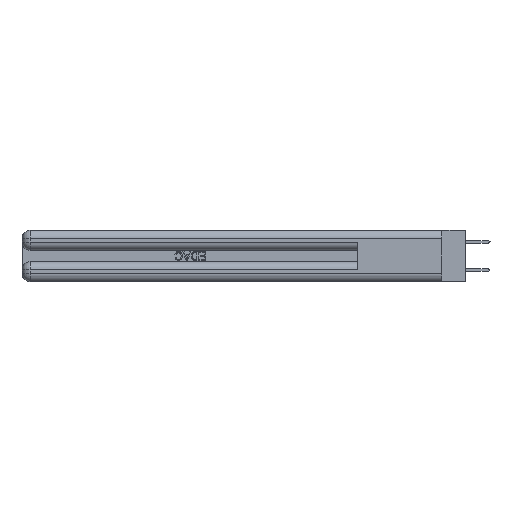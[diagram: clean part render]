
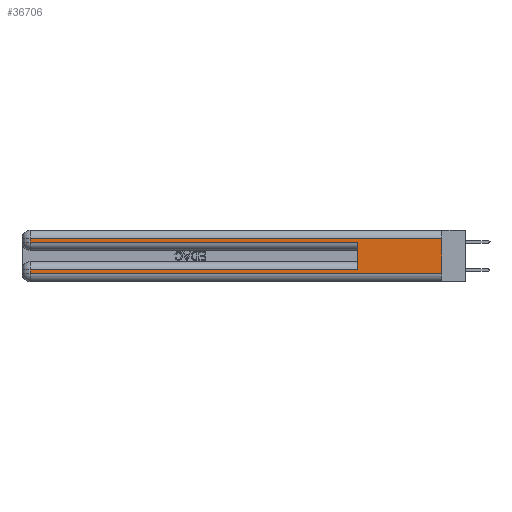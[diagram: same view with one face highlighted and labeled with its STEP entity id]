
A CAD part, left-side view. The second image highlights one B-rep face of the part: STEP entity #36706.
In plain terms, the highlighted planar face has unit normal (-1, 0, 0).
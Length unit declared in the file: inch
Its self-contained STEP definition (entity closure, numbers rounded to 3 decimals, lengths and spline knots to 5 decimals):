
#441 = DIRECTION ( 'NONE',  ( 0., 0., -1. ) ) ;
#700 = CARTESIAN_POINT ( 'NONE',  ( 0., 0., 0.37 ) ) ;
#2287 = VERTEX_POINT ( 'NONE', #32644 ) ;
#2754 = LINE ( 'NONE', #5588, #31531 ) ;
#3658 = ORIENTED_EDGE ( 'NONE', *, *, #20269, .T. ) ;
#3815 = FACE_OUTER_BOUND ( 'NONE', #10392, .T. ) ;
#4210 = PLANE ( 'NONE',  #14571 ) ;
#4632 = EDGE_CURVE ( 'NONE', #31829, #2287, #16413, .T. ) ;
#4650 = ORIENTED_EDGE ( 'NONE', *, *, #26256, .F. ) ;
#5177 = VECTOR ( 'NONE', #441, 39.37008 ) ;
#5443 = LINE ( 'NONE', #10753, #28628 ) ;
#5588 = CARTESIAN_POINT ( 'NONE',  ( 0., 0.6, 0.145 ) ) ;
#5664 = LINE ( 'NONE', #700, #5177 ) ;
#6386 = CARTESIAN_POINT ( 'NONE',  ( 0., 2.94, 0.37 ) ) ;
#6624 = VECTOR ( 'NONE', #23971, 39.37008 ) ;
#6666 = VERTEX_POINT ( 'NONE', #29939 ) ;
#7479 = ORIENTED_EDGE ( 'NONE', *, *, #25581, .T. ) ;
#7856 = VECTOR ( 'NONE', #13585, 39.37008 ) ;
#8448 = CARTESIAN_POINT ( 'NONE',  ( 0., 0., 0.285 ) ) ;
#8641 = EDGE_CURVE ( 'NONE', #6666, #14168, #5443, .T. ) ;
#10198 = CARTESIAN_POINT ( 'NONE',  ( 0., 0., 0.37 ) ) ;
#10392 = EDGE_LOOP ( 'NONE', ( #4650, #13393, #21460, #3658, #15044, #21751, #19445, #7479 ) ) ;
#10753 = CARTESIAN_POINT ( 'NONE',  ( 0., 2.94, 0.37 ) ) ;
#11441 = EDGE_CURVE ( 'NONE', #2287, #20490, #22159, .T. ) ;
#12918 = CARTESIAN_POINT ( 'NONE',  ( 0., 0.6, 0.285 ) ) ;
#13330 = VECTOR ( 'NONE', #35353, 39.37008 ) ;
#13393 = ORIENTED_EDGE ( 'NONE', *, *, #4632, .T. ) ;
#13460 = CARTESIAN_POINT ( 'NONE',  ( 0., 0., 0.085 ) ) ;
#13585 = DIRECTION ( 'NONE',  ( 0., 1., 0. ) ) ;
#13697 = DIRECTION ( 'NONE',  ( 0., 0., -1. ) ) ;
#14168 = VERTEX_POINT ( 'NONE', #26754 ) ;
#14190 = DIRECTION ( 'NONE',  ( 0., -1., 0. ) ) ;
#14571 = AXIS2_PLACEMENT_3D ( 'NONE', #10198, #30933, #25244 ) ;
#15044 = ORIENTED_EDGE ( 'NONE', *, *, #15542, .F. ) ;
#15542 = EDGE_CURVE ( 'NONE', #19315, #20149, #2754, .T. ) ;
#16413 = LINE ( 'NONE', #36492, #27526 ) ;
#16509 = EDGE_CURVE ( 'NONE', #19315, #6666, #22303, .T. ) ;
#16942 = VECTOR ( 'NONE', #14190, 39.37008 ) ;
#18943 = DIRECTION ( 'NONE',  ( 0., 1., 0. ) ) ;
#19315 = VERTEX_POINT ( 'NONE', #35461 ) ;
#19445 = ORIENTED_EDGE ( 'NONE', *, *, #8641, .T. ) ;
#19568 = VERTEX_POINT ( 'NONE', #22042 ) ;
#20149 = VERTEX_POINT ( 'NONE', #12918 ) ;
#20269 = EDGE_CURVE ( 'NONE', #20490, #20149, #28051, .T. ) ;
#20490 = VERTEX_POINT ( 'NONE', #21324 ) ;
#21324 = CARTESIAN_POINT ( 'NONE',  ( 0., 2.94, 0.285 ) ) ;
#21460 = ORIENTED_EDGE ( 'NONE', *, *, #11441, .T. ) ;
#21751 = ORIENTED_EDGE ( 'NONE', *, *, #16509, .T. ) ;
#22042 = CARTESIAN_POINT ( 'NONE',  ( 0., 0., 0.06 ) ) ;
#22159 = LINE ( 'NONE', #6386, #13330 ) ;
#22303 = LINE ( 'NONE', #13460, #7856 ) ;
#23971 = DIRECTION ( 'NONE',  ( 0., -1., 0. ) ) ;
#25244 = DIRECTION ( 'NONE',  ( 0., 0., -1. ) ) ;
#25581 = EDGE_CURVE ( 'NONE', #14168, #19568, #27033, .T. ) ;
#26256 = EDGE_CURVE ( 'NONE', #31829, #19568, #5664, .T. ) ;
#26754 = CARTESIAN_POINT ( 'NONE',  ( 0., 2.94, 0.06 ) ) ;
#27033 = LINE ( 'NONE', #38330, #6624 ) ;
#27526 = VECTOR ( 'NONE', #18943, 39.37008 ) ;
#28051 = LINE ( 'NONE', #8448, #16942 ) ;
#28628 = VECTOR ( 'NONE', #13697, 39.37008 ) ;
#29010 = CARTESIAN_POINT ( 'NONE',  ( 0., 0., 0.31 ) ) ;
#29939 = CARTESIAN_POINT ( 'NONE',  ( 0., 2.94, 0.085 ) ) ;
#30933 = DIRECTION ( 'NONE',  ( 1., 0., 0. ) ) ;
#31531 = VECTOR ( 'NONE', #34976, 39.37008 ) ;
#31829 = VERTEX_POINT ( 'NONE', #29010 ) ;
#32644 = CARTESIAN_POINT ( 'NONE',  ( 0., 2.94, 0.31 ) ) ;
#34976 = DIRECTION ( 'NONE',  ( 0., 0., 1. ) ) ;
#35353 = DIRECTION ( 'NONE',  ( 0., 0., -1. ) ) ;
#35461 = CARTESIAN_POINT ( 'NONE',  ( 0., 0.6, 0.085 ) ) ;
#36492 = CARTESIAN_POINT ( 'NONE',  ( 0., 0., 0.31 ) ) ;
#36706 = ADVANCED_FACE ( 'NONE', ( #3815 ), #4210, .F. ) ;
#38330 = CARTESIAN_POINT ( 'NONE',  ( 0., 0., 0.06 ) ) ;
